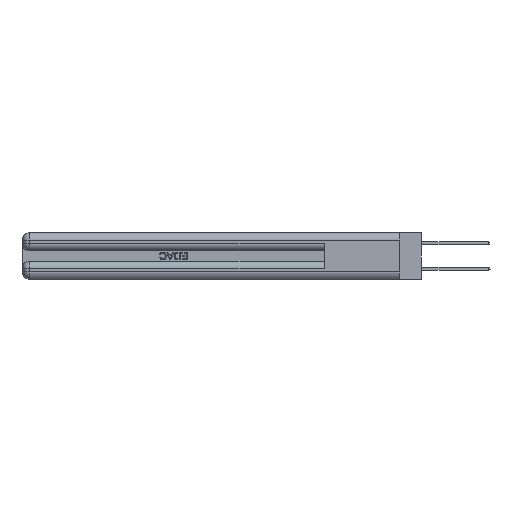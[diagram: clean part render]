
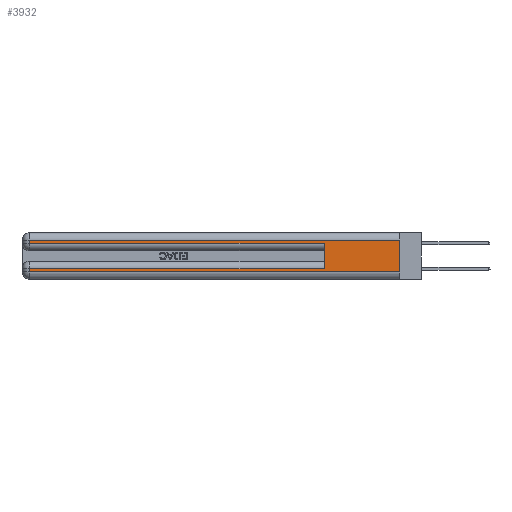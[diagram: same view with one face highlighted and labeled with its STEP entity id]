
A CAD part, left-side view. The second image highlights one B-rep face of the part: STEP entity #3932.
In plain terms, the highlighted planar face has unit normal (-1, 0, 0).
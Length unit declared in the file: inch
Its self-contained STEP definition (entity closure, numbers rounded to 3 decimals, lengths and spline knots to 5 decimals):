
#201 = EDGE_CURVE ( 'NONE', #12714, #26932, #12371, .T. ) ;
#782 = VERTEX_POINT ( 'NONE', #7273 ) ;
#1020 = CARTESIAN_POINT ( 'NONE',  ( 0., 2.94, 0.06 ) ) ;
#1125 = CARTESIAN_POINT ( 'NONE',  ( 0., 0., 0.085 ) ) ;
#1720 = EDGE_CURVE ( 'NONE', #782, #43497, #36072, .T. ) ;
#2644 = ORIENTED_EDGE ( 'NONE', *, *, #16252, .F. ) ;
#3846 = DIRECTION ( 'NONE',  ( 0., 1., 0. ) ) ;
#3932 = ADVANCED_FACE ( 'NONE', ( #41371 ), #43338, .F. ) ;
#5281 = LINE ( 'NONE', #36220, #40867 ) ;
#5815 = LINE ( 'NONE', #10521, #33069 ) ;
#6224 = VERTEX_POINT ( 'NONE', #38527 ) ;
#7273 = CARTESIAN_POINT ( 'NONE',  ( 0., 0.6, 0.085 ) ) ;
#7799 = DIRECTION ( 'NONE',  ( 0., -1., 0. ) ) ;
#8153 = EDGE_CURVE ( 'NONE', #45058, #14752, #14542, .T. ) ;
#8425 = VECTOR ( 'NONE', #24168, 39.37008 ) ;
#10521 = CARTESIAN_POINT ( 'NONE',  ( 0., 0., 0.37 ) ) ;
#10973 = CARTESIAN_POINT ( 'NONE',  ( 0., 0., 0.31 ) ) ;
#10995 = CARTESIAN_POINT ( 'NONE',  ( 0., 0., 0.06 ) ) ;
#11994 = VECTOR ( 'NONE', #3846, 39.37008 ) ;
#12073 = EDGE_CURVE ( 'NONE', #6224, #26932, #5815, .T. ) ;
#12371 = LINE ( 'NONE', #10995, #22947 ) ;
#12714 = VERTEX_POINT ( 'NONE', #1020 ) ;
#14220 = AXIS2_PLACEMENT_3D ( 'NONE', #22189, #39938, #18768 ) ;
#14542 = LINE ( 'NONE', #21807, #32228 ) ;
#14752 = VERTEX_POINT ( 'NONE', #15701 ) ;
#14763 = CARTESIAN_POINT ( 'NONE',  ( 0., 0.6, 0.285 ) ) ;
#15017 = ORIENTED_EDGE ( 'NONE', *, *, #28981, .T. ) ;
#15701 = CARTESIAN_POINT ( 'NONE',  ( 0., 2.94, 0.285 ) ) ;
#16252 = EDGE_CURVE ( 'NONE', #782, #35883, #28439, .T. ) ;
#17244 = VECTOR ( 'NONE', #33127, 39.37008 ) ;
#18768 = DIRECTION ( 'NONE',  ( 0., 0., -1. ) ) ;
#20104 = EDGE_CURVE ( 'NONE', #6224, #45058, #21467, .T. ) ;
#20440 = EDGE_LOOP ( 'NONE', ( #30947, #42594, #24894, #36123, #2644, #21748, #15017, #43240 ) ) ;
#20628 = CARTESIAN_POINT ( 'NONE',  ( 0., 0.6, 0.145 ) ) ;
#21467 = LINE ( 'NONE', #10973, #11994 ) ;
#21748 = ORIENTED_EDGE ( 'NONE', *, *, #1720, .T. ) ;
#21807 = CARTESIAN_POINT ( 'NONE',  ( 0., 2.94, 0.37 ) ) ;
#22189 = CARTESIAN_POINT ( 'NONE',  ( 0., 0., 0.37 ) ) ;
#22947 = VECTOR ( 'NONE', #36962, 39.37008 ) ;
#24168 = DIRECTION ( 'NONE',  ( 0., 0., 1. ) ) ;
#24505 = CARTESIAN_POINT ( 'NONE',  ( 0., 2.94, 0.31 ) ) ;
#24894 = ORIENTED_EDGE ( 'NONE', *, *, #8153, .T. ) ;
#25733 = EDGE_CURVE ( 'NONE', #14752, #35883, #5281, .T. ) ;
#26111 = CARTESIAN_POINT ( 'NONE',  ( 0., 2.94, 0.085 ) ) ;
#26932 = VERTEX_POINT ( 'NONE', #35496 ) ;
#27593 = LINE ( 'NONE', #32178, #35914 ) ;
#28439 = LINE ( 'NONE', #20628, #8425 ) ;
#28807 = DIRECTION ( 'NONE',  ( 0., 0., -1. ) ) ;
#28981 = EDGE_CURVE ( 'NONE', #43497, #12714, #27593, .T. ) ;
#30947 = ORIENTED_EDGE ( 'NONE', *, *, #12073, .F. ) ;
#31747 = DIRECTION ( 'NONE',  ( 0., 0., -1. ) ) ;
#32178 = CARTESIAN_POINT ( 'NONE',  ( 0., 2.94, 0.37 ) ) ;
#32228 = VECTOR ( 'NONE', #32588, 39.37008 ) ;
#32588 = DIRECTION ( 'NONE',  ( 0., 0., -1. ) ) ;
#33069 = VECTOR ( 'NONE', #31747, 39.37008 ) ;
#33127 = DIRECTION ( 'NONE',  ( 0., 1., 0. ) ) ;
#35496 = CARTESIAN_POINT ( 'NONE',  ( 0., 0., 0.06 ) ) ;
#35883 = VERTEX_POINT ( 'NONE', #14763 ) ;
#35914 = VECTOR ( 'NONE', #28807, 39.37008 ) ;
#36072 = LINE ( 'NONE', #1125, #17244 ) ;
#36123 = ORIENTED_EDGE ( 'NONE', *, *, #25733, .T. ) ;
#36220 = CARTESIAN_POINT ( 'NONE',  ( 0., 0., 0.285 ) ) ;
#36962 = DIRECTION ( 'NONE',  ( 0., -1., 0. ) ) ;
#38527 = CARTESIAN_POINT ( 'NONE',  ( 0., 0., 0.31 ) ) ;
#39938 = DIRECTION ( 'NONE',  ( 1., 0., 0. ) ) ;
#40867 = VECTOR ( 'NONE', #7799, 39.37008 ) ;
#41371 = FACE_OUTER_BOUND ( 'NONE', #20440, .T. ) ;
#42594 = ORIENTED_EDGE ( 'NONE', *, *, #20104, .T. ) ;
#43240 = ORIENTED_EDGE ( 'NONE', *, *, #201, .T. ) ;
#43338 = PLANE ( 'NONE',  #14220 ) ;
#43497 = VERTEX_POINT ( 'NONE', #26111 ) ;
#45058 = VERTEX_POINT ( 'NONE', #24505 ) ;
